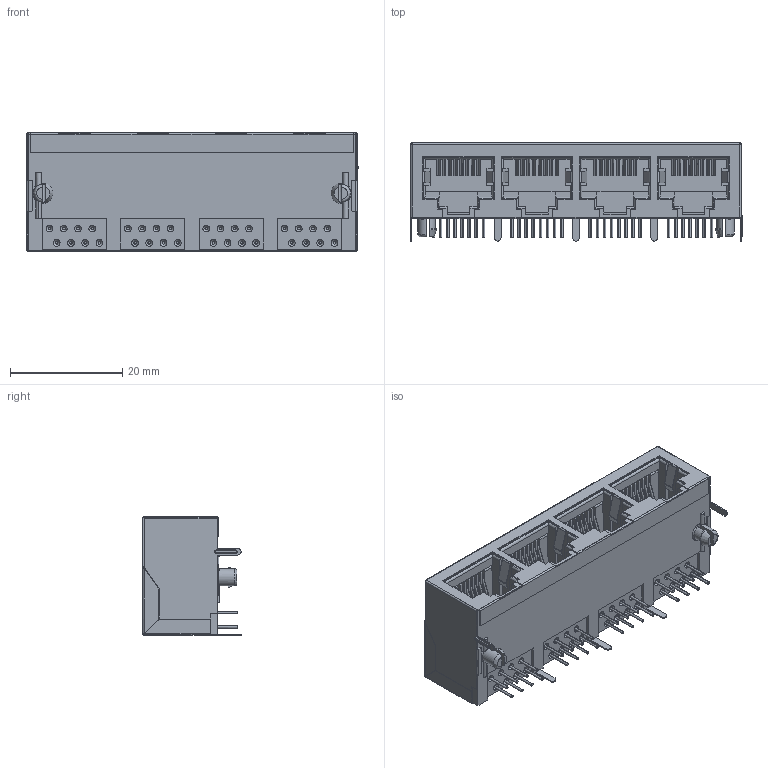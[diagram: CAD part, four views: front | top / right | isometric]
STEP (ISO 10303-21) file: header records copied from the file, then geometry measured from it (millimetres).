
FILE_DESCRIPTION (( 'STEP AP203' ), '1' );
FILE_NAME ('RJ93048822N00101.STEP', '2020-01-20T16:28:14', ( '' ), ( '' ), 'SwSTEP 2.0', 'SolidWorks 2016', '' );
FILE_SCHEMA (( 'CONFIG_CONTROL_DESIGN' ));
Length unit declared in the file: millimetre
Products named in the file (5): 93 Shield; 93 Contact Lock; RJ93048822N00101; 93 Contacts; 93 Insulator
Assembly tree (10 placements, depth 2):
  RJ93048822N00101
    93 Insulator
    93 Contacts  x4
    93 Contact Lock  x4
    93 Shield
Bounding box: 59.2 x 17.5 x 21.14 mm (x, y, z)
Volume: 9684.3 mm3; surface area: 21055.9 mm2
Topology: 38 solids, 38 shells, 2070 faces, 5654 edges, 3686 vertices
Faces by surface type: plane 1065, cylinder 665, bspline 146, torus 128, cone 66
Entity records: 37140 total; most frequent: CARTESIAN_POINT 7753, ORIENTED_EDGE 6244, DIRECTION 5766, EDGE_CURVE 3122, VECTOR 2314, LINE 2314, VERTEX_POINT 2027, AXIS2_PLACEMENT_3D 1726
